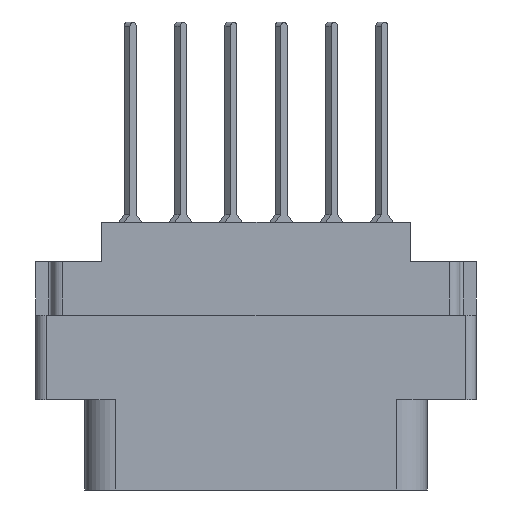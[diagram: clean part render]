
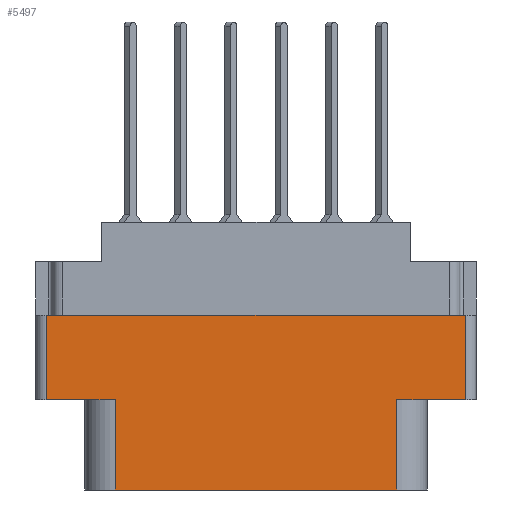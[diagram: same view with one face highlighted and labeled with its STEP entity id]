
A CAD part, front view. The second image highlights one B-rep face of the part: STEP entity #5497.
In plain terms, the highlighted planar face has unit normal (0, -1, 0).
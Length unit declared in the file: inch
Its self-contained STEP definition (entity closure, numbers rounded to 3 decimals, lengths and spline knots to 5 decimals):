
#49 = DIRECTION ( 'NONE',  ( 0., 0., 1. ) ) ;
#225 = VECTOR ( 'NONE', #15615, 39.37008 ) ;
#614 = ORIENTED_EDGE ( 'NONE', *, *, #20918, .F. ) ;
#850 = EDGE_CURVE ( 'NONE', #5770, #16616, #11102, .T. ) ;
#1150 = VECTOR ( 'NONE', #7802, 39.37008 ) ;
#1359 = DIRECTION ( 'NONE',  ( 1., 0., 0. ) ) ;
#1664 = VECTOR ( 'NONE', #1359, 39.37008 ) ;
#1887 = LINE ( 'NONE', #16030, #19663 ) ;
#2166 = VECTOR ( 'NONE', #49, 39.37008 ) ;
#2462 = CARTESIAN_POINT ( 'NONE',  ( 0.42, -0.343, -0.529 ) ) ;
#2734 = ORIENTED_EDGE ( 'NONE', *, *, #18866, .T. ) ;
#2770 = CARTESIAN_POINT ( 'NONE',  ( -0.624, -0.343, -0.529 ) ) ;
#2972 = FACE_OUTER_BOUND ( 'NONE', #13263, .T. ) ;
#2984 = VERTEX_POINT ( 'NONE', #12643 ) ;
#2994 = CARTESIAN_POINT ( 'NONE',  ( 0.624, -0.343, -0.529 ) ) ;
#3408 = DIRECTION ( 'NONE',  ( -1., 0., 0. ) ) ;
#3628 = CARTESIAN_POINT ( 'NONE',  ( 0.42, -0.343, -0.798 ) ) ;
#3893 = LINE ( 'NONE', #2462, #5645 ) ;
#4517 = EDGE_CURVE ( 'NONE', #5770, #19035, #14430, .T. ) ;
#4522 = DIRECTION ( 'NONE',  ( 0., 0., -1. ) ) ;
#4569 = VECTOR ( 'NONE', #4522, 39.37008 ) ;
#4761 = ORIENTED_EDGE ( 'NONE', *, *, #4517, .F. ) ;
#4925 = DIRECTION ( 'NONE',  ( 1., 0., 0. ) ) ;
#5331 = CARTESIAN_POINT ( 'NONE',  ( 0., -0.343, -0.529 ) ) ;
#5467 = AXIS2_PLACEMENT_3D ( 'NONE', #16270, #23714, #12576 ) ;
#5497 = ADVANCED_FACE ( 'NONE', ( #2972 ), #18000, .T. ) ;
#5645 = VECTOR ( 'NONE', #13726, 39.37008 ) ;
#5770 = VERTEX_POINT ( 'NONE', #2770 ) ;
#6052 = VERTEX_POINT ( 'NONE', #12906 ) ;
#6644 = LINE ( 'NONE', #12069, #225 ) ;
#7130 = CARTESIAN_POINT ( 'NONE',  ( -0.624, -0.343, -0.277 ) ) ;
#7308 = VERTEX_POINT ( 'NONE', #3628 ) ;
#7741 = VECTOR ( 'NONE', #3408, 39.37008 ) ;
#7802 = DIRECTION ( 'NONE',  ( 1., 0., 0. ) ) ;
#11102 = LINE ( 'NONE', #17089, #1150 ) ;
#11458 = ORIENTED_EDGE ( 'NONE', *, *, #22275, .T. ) ;
#12069 = CARTESIAN_POINT ( 'NONE',  ( 0.624, -0.343, -0.798 ) ) ;
#12089 = ORIENTED_EDGE ( 'NONE', *, *, #13778, .F. ) ;
#12576 = DIRECTION ( 'NONE',  ( 0., 0., -1. ) ) ;
#12643 = CARTESIAN_POINT ( 'NONE',  ( 0.42, -0.343, -0.529 ) ) ;
#12906 = CARTESIAN_POINT ( 'NONE',  ( 0.624, -0.343, -0.277 ) ) ;
#13263 = EDGE_LOOP ( 'NONE', ( #11458, #2734, #614, #22927, #13992, #12089, #4761, #16386 ) ) ;
#13372 = LINE ( 'NONE', #23394, #4569 ) ;
#13726 = DIRECTION ( 'NONE',  ( 0., 0., -1. ) ) ;
#13778 = EDGE_CURVE ( 'NONE', #19035, #6052, #1887, .T. ) ;
#13992 = ORIENTED_EDGE ( 'NONE', *, *, #17270, .T. ) ;
#14430 = LINE ( 'NONE', #16932, #2166 ) ;
#15615 = DIRECTION ( 'NONE',  ( 0., 0., 1. ) ) ;
#15739 = VERTEX_POINT ( 'NONE', #16789 ) ;
#16030 = CARTESIAN_POINT ( 'NONE',  ( -0.656, -0.343, -0.277 ) ) ;
#16270 = CARTESIAN_POINT ( 'NONE',  ( -0.624, -0.343, -0.798 ) ) ;
#16386 = ORIENTED_EDGE ( 'NONE', *, *, #850, .T. ) ;
#16616 = VERTEX_POINT ( 'NONE', #22995 ) ;
#16789 = CARTESIAN_POINT ( 'NONE',  ( -0.42, -0.343, -0.798 ) ) ;
#16932 = CARTESIAN_POINT ( 'NONE',  ( -0.624, -0.343, -0.798 ) ) ;
#17089 = CARTESIAN_POINT ( 'NONE',  ( 0., -0.343, -0.529 ) ) ;
#17270 = EDGE_CURVE ( 'NONE', #20713, #6052, #6644, .T. ) ;
#18000 = PLANE ( 'NONE',  #5467 ) ;
#18866 = EDGE_CURVE ( 'NONE', #15739, #7308, #19737, .T. ) ;
#19035 = VERTEX_POINT ( 'NONE', #7130 ) ;
#19663 = VECTOR ( 'NONE', #4925, 39.37008 ) ;
#19737 = LINE ( 'NONE', #23712, #1664 ) ;
#20713 = VERTEX_POINT ( 'NONE', #2994 ) ;
#20918 = EDGE_CURVE ( 'NONE', #2984, #7308, #3893, .T. ) ;
#22275 = EDGE_CURVE ( 'NONE', #16616, #15739, #13372, .T. ) ;
#22637 = LINE ( 'NONE', #5331, #7741 ) ;
#22927 = ORIENTED_EDGE ( 'NONE', *, *, #24166, .F. ) ;
#22995 = CARTESIAN_POINT ( 'NONE',  ( -0.42, -0.343, -0.529 ) ) ;
#23394 = CARTESIAN_POINT ( 'NONE',  ( -0.42, -0.343, -0.529 ) ) ;
#23712 = CARTESIAN_POINT ( 'NONE',  ( -0.624, -0.343, -0.798 ) ) ;
#23714 = DIRECTION ( 'NONE',  ( 0., -1., 0. ) ) ;
#24166 = EDGE_CURVE ( 'NONE', #20713, #2984, #22637, .T. ) ;
